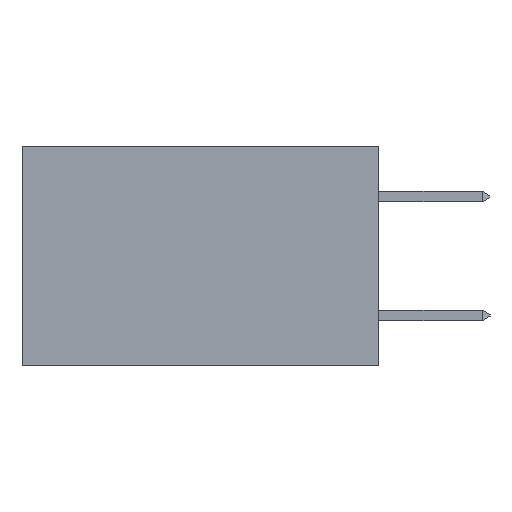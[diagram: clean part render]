
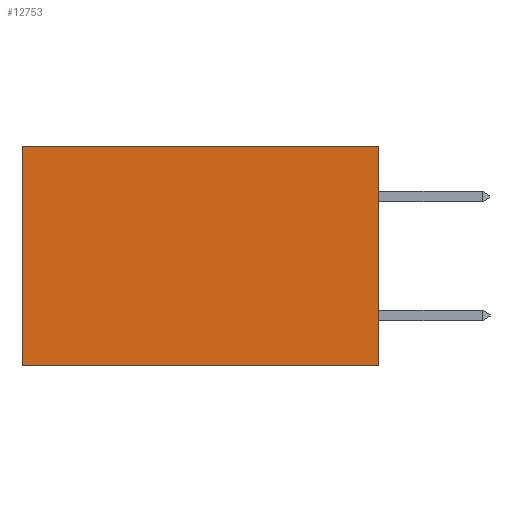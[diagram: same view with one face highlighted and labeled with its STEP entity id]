
A CAD part, left-side view. The second image highlights one B-rep face of the part: STEP entity #12753.
In plain terms, the highlighted planar face has unit normal (-1, 0, 0).
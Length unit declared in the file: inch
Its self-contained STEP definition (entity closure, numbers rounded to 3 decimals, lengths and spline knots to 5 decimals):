
#12 = CARTESIAN_POINT ( 'NONE',  ( 0.2615, 0.6, -0.37 ) ) ;
#506 = CARTESIAN_POINT ( 'NONE',  ( 0.2615, 0.6, 0. ) ) ;
#546 = CARTESIAN_POINT ( 'NONE',  ( 0.2615, 0.6, -0.37 ) ) ;
#551 = DIRECTION ( 'NONE',  ( 0., 0., -1. ) ) ;
#1867 = VECTOR ( 'NONE', #4402, 39.37008 ) ;
#1888 = ORIENTED_EDGE ( 'NONE', *, *, #11278, .T. ) ;
#3685 = VERTEX_POINT ( 'NONE', #4423 ) ;
#3957 = VECTOR ( 'NONE', #6735, 39.37008 ) ;
#4105 = LINE ( 'NONE', #6036, #11763 ) ;
#4199 = DIRECTION ( 'NONE',  ( 1., 0., 0. ) ) ;
#4218 = EDGE_CURVE ( 'NONE', #3685, #9006, #4320, .T. ) ;
#4320 = LINE ( 'NONE', #6887, #3957 ) ;
#4387 = CARTESIAN_POINT ( 'NONE',  ( 0.2615, 0., 0. ) ) ;
#4402 = DIRECTION ( 'NONE',  ( 0., 1., 0. ) ) ;
#4423 = CARTESIAN_POINT ( 'NONE',  ( 0.2615, 0., -0.37 ) ) ;
#5109 = ORIENTED_EDGE ( 'NONE', *, *, #6582, .T. ) ;
#5632 = VECTOR ( 'NONE', #551, 39.37008 ) ;
#5759 = FACE_OUTER_BOUND ( 'NONE', #11779, .T. ) ;
#6006 = DIRECTION ( 'NONE',  ( 0., 0., -1. ) ) ;
#6036 = CARTESIAN_POINT ( 'NONE',  ( 0.2615, 0., -0.37 ) ) ;
#6372 = PLANE ( 'NONE',  #7405 ) ;
#6514 = ORIENTED_EDGE ( 'NONE', *, *, #8355, .F. ) ;
#6582 = EDGE_CURVE ( 'NONE', #11301, #6988, #10145, .T. ) ;
#6735 = DIRECTION ( 'NONE',  ( 0., 1., 0. ) ) ;
#6887 = CARTESIAN_POINT ( 'NONE',  ( 0.2615, 0., -0.37 ) ) ;
#6988 = VERTEX_POINT ( 'NONE', #506 ) ;
#7405 = AXIS2_PLACEMENT_3D ( 'NONE', #10469, #4199, #11487 ) ;
#8355 = EDGE_CURVE ( 'NONE', #11301, #3685, #4105, .T. ) ;
#8423 = LINE ( 'NONE', #546, #5632 ) ;
#9006 = VERTEX_POINT ( 'NONE', #12 ) ;
#10145 = LINE ( 'NONE', #4387, #1867 ) ;
#10469 = CARTESIAN_POINT ( 'NONE',  ( 0.2615, 0., -0.37 ) ) ;
#11153 = ORIENTED_EDGE ( 'NONE', *, *, #4218, .F. ) ;
#11278 = EDGE_CURVE ( 'NONE', #6988, #9006, #8423, .T. ) ;
#11301 = VERTEX_POINT ( 'NONE', #13096 ) ;
#11487 = DIRECTION ( 'NONE',  ( 0., 0., -1. ) ) ;
#11763 = VECTOR ( 'NONE', #6006, 39.37008 ) ;
#11779 = EDGE_LOOP ( 'NONE', ( #1888, #11153, #6514, #5109 ) ) ;
#12753 = ADVANCED_FACE ( 'NONE', ( #5759 ), #6372, .F. ) ;
#13096 = CARTESIAN_POINT ( 'NONE',  ( 0.2615, 0., 0. ) ) ;
